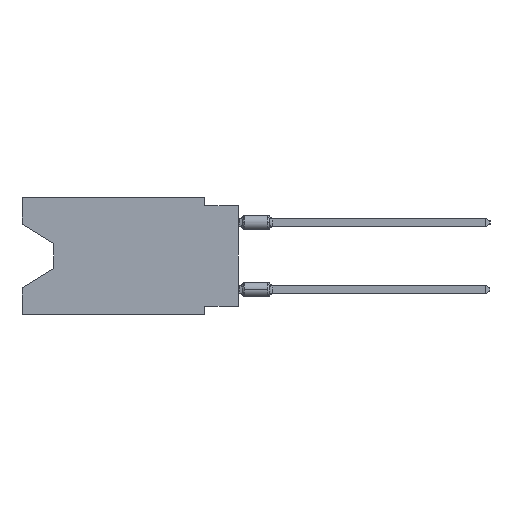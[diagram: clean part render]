
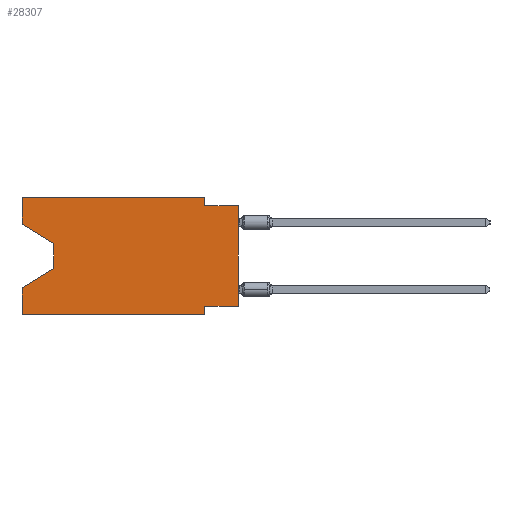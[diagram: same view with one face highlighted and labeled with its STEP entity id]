
A CAD part, left-side view. The second image highlights one B-rep face of the part: STEP entity #28307.
In plain terms, the highlighted planar face has unit normal (-1, 0, 0).
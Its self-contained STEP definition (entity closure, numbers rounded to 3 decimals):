
#190 = VECTOR ( 'NONE', #10170, 1000. ) ;
#425 = DIRECTION ( 'NONE',  ( 0., 0., 1. ) ) ;
#1843 = DIRECTION ( 'NONE',  ( 0., 0., 1. ) ) ;
#2502 = VECTOR ( 'NONE', #6271, 1000. ) ;
#2513 = DIRECTION ( 'NONE',  ( 0., 0., -1. ) ) ;
#3167 = CARTESIAN_POINT ( 'NONE',  ( 0., 0., -0.635 ) ) ;
#3481 = CARTESIAN_POINT ( 'NONE',  ( 0., 2.54, -8.89 ) ) ;
#4050 = CARTESIAN_POINT ( 'NONE',  ( 0., 16.383, -8.89 ) ) ;
#4068 = CARTESIAN_POINT ( 'NONE',  ( 0., 16.383, -2.038 ) ) ;
#4095 = CARTESIAN_POINT ( 'NONE',  ( 0., 16.383, 0. ) ) ;
#4436 = VERTEX_POINT ( 'NONE', #3167 ) ;
#6137 = VECTOR ( 'NONE', #10990, 1000. ) ;
#6271 = DIRECTION ( 'NONE',  ( 0., -1., 0. ) ) ;
#6477 = ORIENTED_EDGE ( 'NONE', *, *, #18016, .F. ) ;
#6631 = VECTOR ( 'NONE', #1843, 1000. ) ;
#6643 = FACE_OUTER_BOUND ( 'NONE', #46480, .T. ) ;
#6723 = CARTESIAN_POINT ( 'NONE',  ( 0., 2.54, 0. ) ) ;
#6839 = VECTOR ( 'NONE', #425, 1000. ) ;
#10170 = DIRECTION ( 'NONE',  ( 0., -1., 0. ) ) ;
#10876 = ORIENTED_EDGE ( 'NONE', *, *, #29620, .F. ) ;
#10990 = DIRECTION ( 'NONE',  ( 0., 0., -1. ) ) ;
#11067 = CARTESIAN_POINT ( 'NONE',  ( 0., 16.383, 0. ) ) ;
#11694 = DIRECTION ( 'NONE',  ( 0., -0.855, -0.519 ) ) ;
#11935 = DIRECTION ( 'NONE',  ( 1., 0., 0. ) ) ;
#12702 = ORIENTED_EDGE ( 'NONE', *, *, #54363, .T. ) ;
#13012 = LINE ( 'NONE', #34263, #51487 ) ;
#13865 = CARTESIAN_POINT ( 'NONE',  ( 0., 16.383, -6.852 ) ) ;
#14221 = CARTESIAN_POINT ( 'NONE',  ( 0., 16.383, -8.89 ) ) ;
#15057 = CARTESIAN_POINT ( 'NONE',  ( 0., 2.54, -8.255 ) ) ;
#16121 = CARTESIAN_POINT ( 'NONE',  ( 0., 16.383, 0. ) ) ;
#16972 = CARTESIAN_POINT ( 'NONE',  ( 0., 0., 0. ) ) ;
#18016 = EDGE_CURVE ( 'NONE', #49175, #22994, #40150, .T. ) ;
#18453 = ORIENTED_EDGE ( 'NONE', *, *, #37309, .F. ) ;
#18590 = LINE ( 'NONE', #22792, #2502 ) ;
#19498 = PLANE ( 'NONE',  #25693 ) ;
#19535 = VERTEX_POINT ( 'NONE', #38047 ) ;
#21109 = DIRECTION ( 'NONE',  ( 0., -1., 0. ) ) ;
#21382 = LINE ( 'NONE', #4050, #47976 ) ;
#22188 = VERTEX_POINT ( 'NONE', #52844 ) ;
#22792 = CARTESIAN_POINT ( 'NONE',  ( 0., 16.383, 0. ) ) ;
#22994 = VERTEX_POINT ( 'NONE', #13865 ) ;
#23854 = CARTESIAN_POINT ( 'NONE',  ( 0., 13.97, -3.505 ) ) ;
#23976 = DIRECTION ( 'NONE',  ( 0., 0., -1. ) ) ;
#24631 = ORIENTED_EDGE ( 'NONE', *, *, #41448, .T. ) ;
#24777 = EDGE_CURVE ( 'NONE', #43862, #4436, #28070, .T. ) ;
#25235 = VERTEX_POINT ( 'NONE', #33557 ) ;
#25317 = LINE ( 'NONE', #34812, #6839 ) ;
#25693 = AXIS2_PLACEMENT_3D ( 'NONE', #16121, #11935, #23976 ) ;
#28000 = LINE ( 'NONE', #6723, #54365 ) ;
#28070 = LINE ( 'NONE', #40636, #190 ) ;
#28307 = ADVANCED_FACE ( 'NONE', ( #6643 ), #19498, .F. ) ;
#29149 = EDGE_CURVE ( 'NONE', #19535, #25235, #40350, .T. ) ;
#29620 = EDGE_CURVE ( 'NONE', #22188, #43862, #28000, .T. ) ;
#29896 = VERTEX_POINT ( 'NONE', #43312 ) ;
#30135 = DIRECTION ( 'NONE',  ( 0., 0., 1. ) ) ;
#33524 = CARTESIAN_POINT ( 'NONE',  ( 0., 13.97, -5.385 ) ) ;
#33557 = CARTESIAN_POINT ( 'NONE',  ( 0., 13.97, -5.385 ) ) ;
#33962 = DIRECTION ( 'NONE',  ( 0., 0., -1. ) ) ;
#34263 = CARTESIAN_POINT ( 'NONE',  ( 0., 0., -8.255 ) ) ;
#34760 = EDGE_CURVE ( 'NONE', #25235, #22994, #50561, .T. ) ;
#34812 = CARTESIAN_POINT ( 'NONE',  ( 0., 16.383, 0. ) ) ;
#36084 = VECTOR ( 'NONE', #11694, 1000. ) ;
#36153 = EDGE_CURVE ( 'NONE', #49175, #49783, #21382, .T. ) ;
#37065 = CARTESIAN_POINT ( 'NONE',  ( 0., 2.54, -8.89 ) ) ;
#37289 = EDGE_CURVE ( 'NONE', #29896, #43190, #25317, .T. ) ;
#37309 = EDGE_CURVE ( 'NONE', #47391, #50597, #13012, .T. ) ;
#37727 = CARTESIAN_POINT ( 'NONE',  ( 0., 2.54, -0.635 ) ) ;
#37987 = DIRECTION ( 'NONE',  ( 0., 0.855, -0.519 ) ) ;
#38047 = CARTESIAN_POINT ( 'NONE',  ( 0., 13.97, -3.505 ) ) ;
#38235 = LINE ( 'NONE', #16972, #41974 ) ;
#38760 = EDGE_CURVE ( 'NONE', #43190, #22188, #18590, .T. ) ;
#40150 = LINE ( 'NONE', #11067, #6631 ) ;
#40350 = LINE ( 'NONE', #23854, #6137 ) ;
#40636 = CARTESIAN_POINT ( 'NONE',  ( 0., 0., -0.635 ) ) ;
#41448 = EDGE_CURVE ( 'NONE', #29896, #19535, #49988, .T. ) ;
#41974 = VECTOR ( 'NONE', #30135, 1000. ) ;
#42351 = LINE ( 'NONE', #3481, #48283 ) ;
#42366 = DIRECTION ( 'NONE',  ( 0., 1., 0. ) ) ;
#43190 = VERTEX_POINT ( 'NONE', #4095 ) ;
#43312 = CARTESIAN_POINT ( 'NONE',  ( 0., 16.383, -2.038 ) ) ;
#43862 = VERTEX_POINT ( 'NONE', #37727 ) ;
#44722 = ORIENTED_EDGE ( 'NONE', *, *, #24777, .F. ) ;
#46058 = VECTOR ( 'NONE', #37987, 1000. ) ;
#46480 = EDGE_LOOP ( 'NONE', ( #24631, #46979, #51075, #6477, #46898, #52347, #18453, #12702, #44722, #10876, #47404, #46681 ) ) ;
#46681 = ORIENTED_EDGE ( 'NONE', *, *, #37289, .F. ) ;
#46898 = ORIENTED_EDGE ( 'NONE', *, *, #36153, .T. ) ;
#46979 = ORIENTED_EDGE ( 'NONE', *, *, #29149, .T. ) ;
#47391 = VERTEX_POINT ( 'NONE', #49280 ) ;
#47404 = ORIENTED_EDGE ( 'NONE', *, *, #38760, .F. ) ;
#47976 = VECTOR ( 'NONE', #21109, 1000. ) ;
#48283 = VECTOR ( 'NONE', #33962, 1000. ) ;
#49175 = VERTEX_POINT ( 'NONE', #14221 ) ;
#49280 = CARTESIAN_POINT ( 'NONE',  ( 0., 0., -8.255 ) ) ;
#49783 = VERTEX_POINT ( 'NONE', #37065 ) ;
#49896 = EDGE_CURVE ( 'NONE', #50597, #49783, #42351, .T. ) ;
#49988 = LINE ( 'NONE', #4068, #36084 ) ;
#50561 = LINE ( 'NONE', #33524, #46058 ) ;
#50597 = VERTEX_POINT ( 'NONE', #15057 ) ;
#51075 = ORIENTED_EDGE ( 'NONE', *, *, #34760, .T. ) ;
#51487 = VECTOR ( 'NONE', #42366, 1000. ) ;
#52347 = ORIENTED_EDGE ( 'NONE', *, *, #49896, .F. ) ;
#52844 = CARTESIAN_POINT ( 'NONE',  ( 0., 2.54, 0. ) ) ;
#54363 = EDGE_CURVE ( 'NONE', #47391, #4436, #38235, .T. ) ;
#54365 = VECTOR ( 'NONE', #2513, 1000. ) ;
